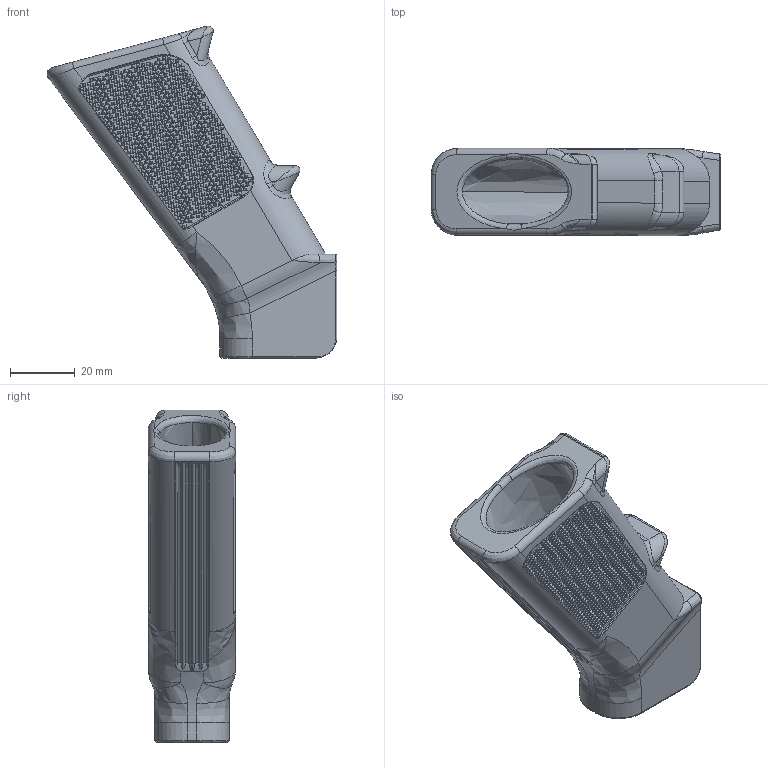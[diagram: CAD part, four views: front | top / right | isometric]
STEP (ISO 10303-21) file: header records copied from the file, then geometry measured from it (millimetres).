
FILE_DESCRIPTION (( 'STEP AP214' ), '1' );
FILE_NAME ('Thunderbolt_Pistol_Grip.STEP', '2021-09-12T03:50:51', ( '' ), ( '' ), 'SwSTEP 2.0', 'SolidWorks 2020', '' );
FILE_SCHEMA (( 'AUTOMOTIVE_DESIGN' ));
Length unit declared in the file: millimetre
Products named in the file (1): Thunderbolt_Pistol_Grip
Bounding box: 89.18 x 26.8 x 102.17 mm (x, y, z)
Volume: 57529.6 mm3; surface area: 24367.8 mm2
Topology: 1 solids, 1 shells, 6189 faces, 12487 edges, 7790 vertices
Faces by surface type: plane 6025, bspline 84, cylinder 80
Entity records: 166018 total; most frequent: CARTESIAN_POINT 43733, ORIENTED_EDGE 24960, DIRECTION 21546, EDGE_CURVE 12480, LINE 9140, VECTOR 9140, VERTEX_POINT 7790, EDGE_LOOP 7688
